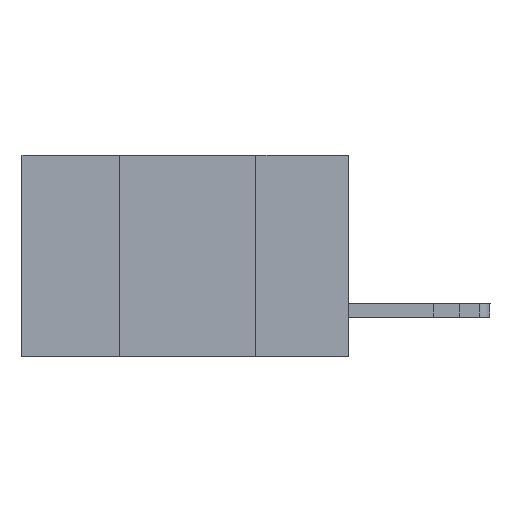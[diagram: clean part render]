
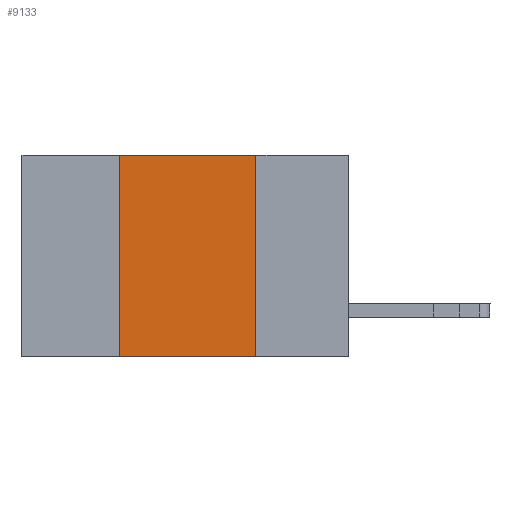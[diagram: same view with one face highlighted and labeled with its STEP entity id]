
A CAD part, left-side view. The second image highlights one B-rep face of the part: STEP entity #9133.
In plain terms, the highlighted planar face has unit normal (-1, 0, 0).
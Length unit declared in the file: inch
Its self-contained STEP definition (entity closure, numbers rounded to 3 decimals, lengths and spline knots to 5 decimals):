
#312 = LINE ( 'NONE', #10933, #4210 ) ;
#932 = EDGE_CURVE ( 'NONE', #7211, #1396, #312, .T. ) ;
#1012 = CARTESIAN_POINT ( 'NONE',  ( 0., 0.6, -0.37 ) ) ;
#1396 = VERTEX_POINT ( 'NONE', #16284 ) ;
#1422 = DIRECTION ( 'NONE',  ( 0., -1., 0. ) ) ;
#1983 = DIRECTION ( 'NONE',  ( 0., 0., 1. ) ) ;
#2366 = DIRECTION ( 'NONE',  ( 1., 0., 0. ) ) ;
#2822 = ORIENTED_EDGE ( 'NONE', *, *, #3915, .F. ) ;
#3353 = CARTESIAN_POINT ( 'NONE',  ( 0., 0.17, 0. ) ) ;
#3915 = EDGE_CURVE ( 'NONE', #1396, #16068, #6637, .T. ) ;
#3920 = ORIENTED_EDGE ( 'NONE', *, *, #932, .F. ) ;
#4055 = DIRECTION ( 'NONE',  ( 0., 0., -1. ) ) ;
#4106 = ORIENTED_EDGE ( 'NONE', *, *, #11760, .F. ) ;
#4210 = VECTOR ( 'NONE', #1983, 39.37008 ) ;
#5191 = VECTOR ( 'NONE', #1422, 39.37008 ) ;
#6637 = LINE ( 'NONE', #11945, #5191 ) ;
#7211 = VERTEX_POINT ( 'NONE', #10729 ) ;
#7375 = DIRECTION ( 'NONE',  ( 0., -1., 0. ) ) ;
#7383 = VERTEX_POINT ( 'NONE', #11756 ) ;
#7743 = CARTESIAN_POINT ( 'NONE',  ( 0., 0.6, 0. ) ) ;
#8151 = LINE ( 'NONE', #15963, #8568 ) ;
#8234 = LINE ( 'NONE', #1012, #12869 ) ;
#8568 = VECTOR ( 'NONE', #4055, 39.37008 ) ;
#9133 = ADVANCED_FACE ( 'NONE', ( #17023 ), #14343, .F. ) ;
#10729 = CARTESIAN_POINT ( 'NONE',  ( 0., 0.42, -0.37 ) ) ;
#10933 = CARTESIAN_POINT ( 'NONE',  ( 0., 0.42, 0. ) ) ;
#11645 = AXIS2_PLACEMENT_3D ( 'NONE', #7743, #2366, #15813 ) ;
#11756 = CARTESIAN_POINT ( 'NONE',  ( 0., 0.17, -0.37 ) ) ;
#11760 = EDGE_CURVE ( 'NONE', #16068, #7383, #8151, .T. ) ;
#11945 = CARTESIAN_POINT ( 'NONE',  ( 0., 0.6, 0. ) ) ;
#12869 = VECTOR ( 'NONE', #7375, 39.37008 ) ;
#14343 = PLANE ( 'NONE',  #11645 ) ;
#15626 = EDGE_CURVE ( 'NONE', #7211, #7383, #8234, .T. ) ;
#15813 = DIRECTION ( 'NONE',  ( 0., 0., -1. ) ) ;
#15816 = EDGE_LOOP ( 'NONE', ( #4106, #2822, #3920, #16551 ) ) ;
#15963 = CARTESIAN_POINT ( 'NONE',  ( 0., 0.17, 0. ) ) ;
#16068 = VERTEX_POINT ( 'NONE', #3353 ) ;
#16284 = CARTESIAN_POINT ( 'NONE',  ( 0., 0.42, 0. ) ) ;
#16551 = ORIENTED_EDGE ( 'NONE', *, *, #15626, .T. ) ;
#17023 = FACE_OUTER_BOUND ( 'NONE', #15816, .T. ) ;
